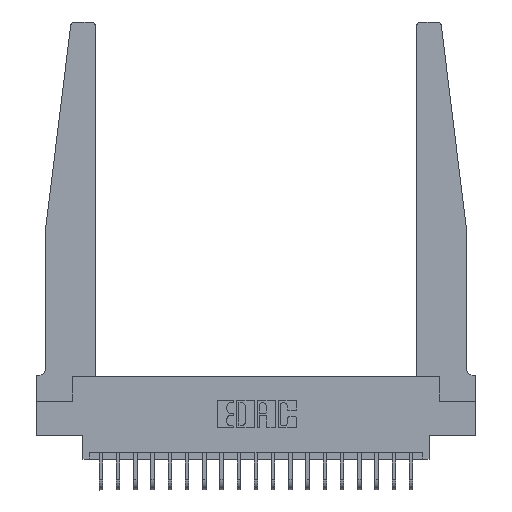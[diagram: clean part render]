
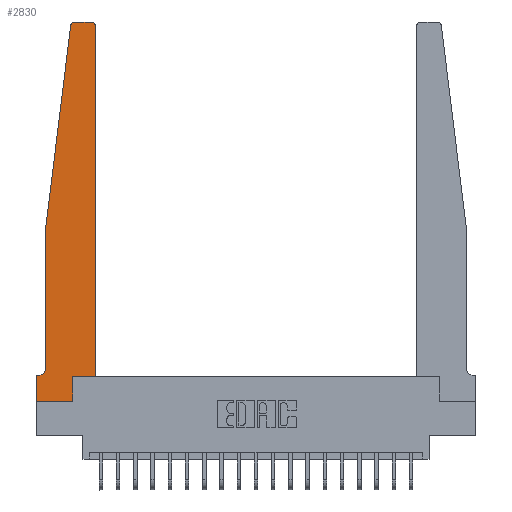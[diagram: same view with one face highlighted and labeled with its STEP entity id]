
A CAD part, top view. The second image highlights one B-rep face of the part: STEP entity #2830.
In plain terms, the highlighted planar face has unit normal (0, 0, 1).
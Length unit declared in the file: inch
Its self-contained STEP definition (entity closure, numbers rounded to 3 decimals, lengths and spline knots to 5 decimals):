
#324 = CIRCLE ( 'NONE', #4343, 0.03 ) ;
#426 = DIRECTION ( 'NONE',  ( 0., -1., 0. ) ) ;
#537 = VERTEX_POINT ( 'NONE', #15194 ) ;
#570 = DIRECTION ( 'NONE',  ( 1., 0., 0. ) ) ;
#652 = LINE ( 'NONE', #10838, #20757 ) ;
#1262 = DIRECTION ( 'NONE',  ( -1., 0., 0. ) ) ;
#1907 = CARTESIAN_POINT ( 'NONE',  ( 0.2605, 0.18, 0.37 ) ) ;
#2187 = ORIENTED_EDGE ( 'NONE', *, *, #6211, .T. ) ;
#2414 = CARTESIAN_POINT ( 'NONE',  ( 0.425, 0.18, 0.37 ) ) ;
#2830 = ADVANCED_FACE ( 'NONE', ( #11925 ), #8158, .T. ) ;
#2855 = DIRECTION ( 'NONE',  ( 0., 0., 1. ) ) ;
#3082 = ORIENTED_EDGE ( 'NONE', *, *, #6062, .T. ) ;
#3088 = ORIENTED_EDGE ( 'NONE', *, *, #12455, .T. ) ;
#3093 = DIRECTION ( 'NONE',  ( 0., 1., 0. ) ) ;
#3214 = EDGE_CURVE ( 'NONE', #537, #13214, #20365, .T. ) ;
#3275 = ORIENTED_EDGE ( 'NONE', *, *, #21635, .T. ) ;
#3405 = LINE ( 'NONE', #20464, #16739 ) ;
#3582 = ORIENTED_EDGE ( 'NONE', *, *, #3780, .T. ) ;
#3780 = EDGE_CURVE ( 'NONE', #6285, #12275, #8187, .T. ) ;
#3971 = ORIENTED_EDGE ( 'NONE', *, *, #20224, .T. ) ;
#4313 = CARTESIAN_POINT ( 'NONE',  ( 0., 0.1875, 0.37 ) ) ;
#4317 = AXIS2_PLACEMENT_3D ( 'NONE', #4704, #16834, #1262 ) ;
#4323 = CARTESIAN_POINT ( 'NONE',  ( 0.065, 1.25, 0.37 ) ) ;
#4343 = AXIS2_PLACEMENT_3D ( 'NONE', #18540, #2855, #570 ) ;
#4352 = CARTESIAN_POINT ( 'NONE',  ( 0.2605, 0.18, 0.37 ) ) ;
#4704 = CARTESIAN_POINT ( 'NONE',  ( 0.015, 0.2375, 0.37 ) ) ;
#5650 = AXIS2_PLACEMENT_3D ( 'NONE', #14909, #9980, #10089 ) ;
#5932 = DIRECTION ( 'NONE',  ( -0.122, -0.992, 0. ) ) ;
#6062 = EDGE_CURVE ( 'NONE', #12275, #537, #16117, .T. ) ;
#6092 = EDGE_CURVE ( 'NONE', #12133, #8509, #652, .T. ) ;
#6184 = DIRECTION ( 'NONE',  ( 1., 0., 0. ) ) ;
#6211 = EDGE_CURVE ( 'NONE', #17577, #11812, #7861, .T. ) ;
#6285 = VERTEX_POINT ( 'NONE', #4313 ) ;
#7139 = CARTESIAN_POINT ( 'NONE',  ( 0.065, 0.2375, 0.37 ) ) ;
#7451 = CARTESIAN_POINT ( 'NONE',  ( 0.425, 2.72, 0.37 ) ) ;
#7551 = EDGE_CURVE ( 'NONE', #14617, #18532, #324, .T. ) ;
#7853 = CARTESIAN_POINT ( 'NONE',  ( 0.25, 2.75, 0.37 ) ) ;
#7861 = LINE ( 'NONE', #9691, #9783 ) ;
#8124 = ORIENTED_EDGE ( 'NONE', *, *, #20850, .T. ) ;
#8158 = PLANE ( 'NONE',  #5650 ) ;
#8187 = LINE ( 'NONE', #21934, #12650 ) ;
#8480 = CARTESIAN_POINT ( 'NONE',  ( 0.065, 1.25, 0.37 ) ) ;
#8509 = VERTEX_POINT ( 'NONE', #7139 ) ;
#9249 = VECTOR ( 'NONE', #15072, 39.37008 ) ;
#9547 = CARTESIAN_POINT ( 'NONE',  ( 0.015, 0.1875, 0.37 ) ) ;
#9603 = EDGE_CURVE ( 'NONE', #18532, #12133, #12809, .T. ) ;
#9691 = CARTESIAN_POINT ( 'NONE',  ( 0.425, 0.18, 0.37 ) ) ;
#9783 = VECTOR ( 'NONE', #13247, 39.37008 ) ;
#9971 = ORIENTED_EDGE ( 'NONE', *, *, #3214, .T. ) ;
#9980 = DIRECTION ( 'NONE',  ( 0., 0., 1. ) ) ;
#10089 = DIRECTION ( 'NONE',  ( 1., 0., 0. ) ) ;
#10838 = CARTESIAN_POINT ( 'NONE',  ( 0.065, 1.25, 0.37 ) ) ;
#11070 = DIRECTION ( 'NONE',  ( 1., 0., 0. ) ) ;
#11180 = CARTESIAN_POINT ( 'NONE',  ( 0., 0., 0.37 ) ) ;
#11750 = CARTESIAN_POINT ( 'NONE',  ( 0.24675, 2.72367, 0.37 ) ) ;
#11812 = VERTEX_POINT ( 'NONE', #7451 ) ;
#11925 = FACE_OUTER_BOUND ( 'NONE', #12164, .T. ) ;
#12122 = AXIS2_PLACEMENT_3D ( 'NONE', #13395, #21870, #6184 ) ;
#12133 = VERTEX_POINT ( 'NONE', #8480 ) ;
#12164 = EDGE_LOOP ( 'NONE', ( #3275, #21512, #13642, #18582, #8124, #20982, #3582, #3082, #9971, #3971, #2187, #3088 ) ) ;
#12275 = VERTEX_POINT ( 'NONE', #12607 ) ;
#12372 = CIRCLE ( 'NONE', #4317, 0.05 ) ;
#12455 = EDGE_CURVE ( 'NONE', #11812, #18105, #15418, .T. ) ;
#12607 = CARTESIAN_POINT ( 'NONE',  ( 0., 0., 0.37 ) ) ;
#12650 = VECTOR ( 'NONE', #12995, 39.37008 ) ;
#12809 = LINE ( 'NONE', #4323, #16063 ) ;
#12995 = DIRECTION ( 'NONE',  ( 0., -1., 0. ) ) ;
#13214 = VERTEX_POINT ( 'NONE', #1907 ) ;
#13247 = DIRECTION ( 'NONE',  ( 0., 1., 0. ) ) ;
#13395 = CARTESIAN_POINT ( 'NONE',  ( 0.395, 2.72, 0.37 ) ) ;
#13578 = CARTESIAN_POINT ( 'NONE',  ( 0.27653, 2.75, 0.37 ) ) ;
#13642 = ORIENTED_EDGE ( 'NONE', *, *, #9603, .T. ) ;
#14133 = CARTESIAN_POINT ( 'NONE',  ( 0.065, 0.1875, 0.37 ) ) ;
#14617 = VERTEX_POINT ( 'NONE', #13578 ) ;
#14851 = VERTEX_POINT ( 'NONE', #9547 ) ;
#14909 = CARTESIAN_POINT ( 'NONE',  ( 0., 0.1875, 0.37 ) ) ;
#15072 = DIRECTION ( 'NONE',  ( -1., 0., 0. ) ) ;
#15194 = CARTESIAN_POINT ( 'NONE',  ( 0.2605, 0., 0.37 ) ) ;
#15418 = CIRCLE ( 'NONE', #12122, 0.03 ) ;
#15547 = DIRECTION ( 'NONE',  ( 1., 0., 0. ) ) ;
#15998 = VECTOR ( 'NONE', #11070, 39.37008 ) ;
#16063 = VECTOR ( 'NONE', #5932, 39.37008 ) ;
#16117 = LINE ( 'NONE', #11180, #15998 ) ;
#16739 = VECTOR ( 'NONE', #15547, 39.37008 ) ;
#16834 = DIRECTION ( 'NONE',  ( 0., 0., -1. ) ) ;
#17577 = VERTEX_POINT ( 'NONE', #2414 ) ;
#17675 = DIRECTION ( 'NONE',  ( -1., 0., 0. ) ) ;
#17906 = LINE ( 'NONE', #14133, #21561 ) ;
#18105 = VERTEX_POINT ( 'NONE', #19901 ) ;
#18532 = VERTEX_POINT ( 'NONE', #11750 ) ;
#18540 = CARTESIAN_POINT ( 'NONE',  ( 0.27653, 2.72, 0.37 ) ) ;
#18582 = ORIENTED_EDGE ( 'NONE', *, *, #6092, .T. ) ;
#18619 = LINE ( 'NONE', #7853, #9249 ) ;
#19901 = CARTESIAN_POINT ( 'NONE',  ( 0.395, 2.75, 0.37 ) ) ;
#20224 = EDGE_CURVE ( 'NONE', #13214, #17577, #3405, .T. ) ;
#20365 = LINE ( 'NONE', #4352, #21392 ) ;
#20464 = CARTESIAN_POINT ( 'NONE',  ( 0.425, 0.18, 0.37 ) ) ;
#20757 = VECTOR ( 'NONE', #426, 39.37008 ) ;
#20850 = EDGE_CURVE ( 'NONE', #8509, #14851, #12372, .T. ) ;
#20982 = ORIENTED_EDGE ( 'NONE', *, *, #21876, .T. ) ;
#21392 = VECTOR ( 'NONE', #3093, 39.37008 ) ;
#21512 = ORIENTED_EDGE ( 'NONE', *, *, #7551, .T. ) ;
#21561 = VECTOR ( 'NONE', #17675, 39.37008 ) ;
#21635 = EDGE_CURVE ( 'NONE', #18105, #14617, #18619, .T. ) ;
#21870 = DIRECTION ( 'NONE',  ( 0., 0., 1. ) ) ;
#21876 = EDGE_CURVE ( 'NONE', #14851, #6285, #17906, .T. ) ;
#21934 = CARTESIAN_POINT ( 'NONE',  ( 0., 0., 0.37 ) ) ;
